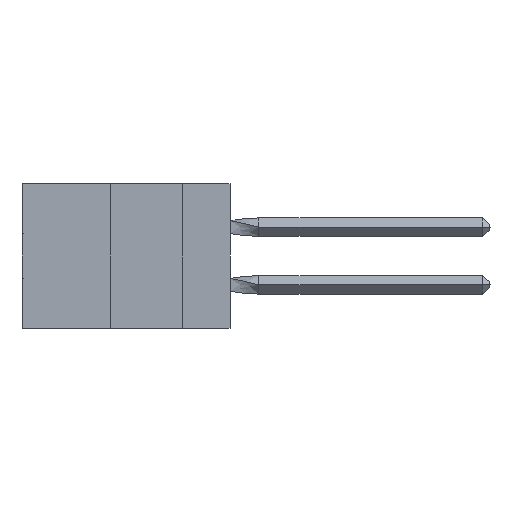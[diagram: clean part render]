
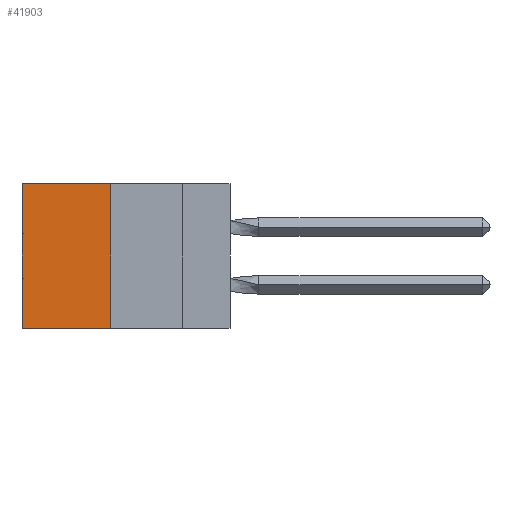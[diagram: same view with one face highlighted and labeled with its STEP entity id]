
A CAD part, left-side view. The second image highlights one B-rep face of the part: STEP entity #41903.
In plain terms, the highlighted planar face has unit normal (-1, 0, 0).
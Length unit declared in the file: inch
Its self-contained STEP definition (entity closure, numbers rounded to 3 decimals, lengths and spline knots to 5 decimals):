
#1044 = ORIENTED_EDGE ( 'NONE', *, *, #18752, .T. ) ;
#1487 = CARTESIAN_POINT ( 'NONE',  ( 0.305, 0.72, 0. ) ) ;
#2749 = VERTEX_POINT ( 'NONE', #1487 ) ;
#3461 = EDGE_CURVE ( 'NONE', #3944, #2749, #13960, .T. ) ;
#3679 = DIRECTION ( 'NONE',  ( 0., 1., 0. ) ) ;
#3944 = VERTEX_POINT ( 'NONE', #40875 ) ;
#4480 = EDGE_CURVE ( 'NONE', #3944, #36482, #26154, .T. ) ;
#7381 = DIRECTION ( 'NONE',  ( 0., 0., -1. ) ) ;
#10095 = PLANE ( 'NONE',  #24794 ) ;
#10259 = EDGE_LOOP ( 'NONE', ( #1044, #18160, #25261, #40814 ) ) ;
#10356 = LINE ( 'NONE', #14954, #35961 ) ;
#10615 = DIRECTION ( 'NONE',  ( 0., 0., -1. ) ) ;
#12928 = LINE ( 'NONE', #33145, #29317 ) ;
#13467 = CARTESIAN_POINT ( 'NONE',  ( 0.305, 0.413, -0.5 ) ) ;
#13542 = DIRECTION ( 'NONE',  ( 1., 0., 0. ) ) ;
#13960 = LINE ( 'NONE', #15164, #30339 ) ;
#14954 = CARTESIAN_POINT ( 'NONE',  ( 0.305, 0.413, -0.5 ) ) ;
#15164 = CARTESIAN_POINT ( 'NONE',  ( 0.305, 0.413, 0. ) ) ;
#18160 = ORIENTED_EDGE ( 'NONE', *, *, #30766, .F. ) ;
#18752 = EDGE_CURVE ( 'NONE', #2749, #23617, #12928, .T. ) ;
#20175 = DIRECTION ( 'NONE',  ( 0., 0., -1. ) ) ;
#23617 = VERTEX_POINT ( 'NONE', #29575 ) ;
#24794 = AXIS2_PLACEMENT_3D ( 'NONE', #36579, #13542, #7381 ) ;
#25261 = ORIENTED_EDGE ( 'NONE', *, *, #4480, .F. ) ;
#26154 = LINE ( 'NONE', #13467, #37938 ) ;
#29317 = VECTOR ( 'NONE', #20175, 39.37008 ) ;
#29575 = CARTESIAN_POINT ( 'NONE',  ( 0.305, 0.72, -0.5 ) ) ;
#30339 = VECTOR ( 'NONE', #38008, 39.37008 ) ;
#30766 = EDGE_CURVE ( 'NONE', #36482, #23617, #10356, .T. ) ;
#32937 = CARTESIAN_POINT ( 'NONE',  ( 0.305, 0.413, -0.5 ) ) ;
#33145 = CARTESIAN_POINT ( 'NONE',  ( 0.305, 0.72, -0.5 ) ) ;
#35961 = VECTOR ( 'NONE', #3679, 39.37008 ) ;
#36482 = VERTEX_POINT ( 'NONE', #32937 ) ;
#36579 = CARTESIAN_POINT ( 'NONE',  ( 0.305, 0.413, -0.5 ) ) ;
#37938 = VECTOR ( 'NONE', #10615, 39.37008 ) ;
#38008 = DIRECTION ( 'NONE',  ( 0., 1., 0. ) ) ;
#39826 = FACE_OUTER_BOUND ( 'NONE', #10259, .T. ) ;
#40814 = ORIENTED_EDGE ( 'NONE', *, *, #3461, .T. ) ;
#40875 = CARTESIAN_POINT ( 'NONE',  ( 0.305, 0.413, 0. ) ) ;
#41903 = ADVANCED_FACE ( 'NONE', ( #39826 ), #10095, .F. ) ;
